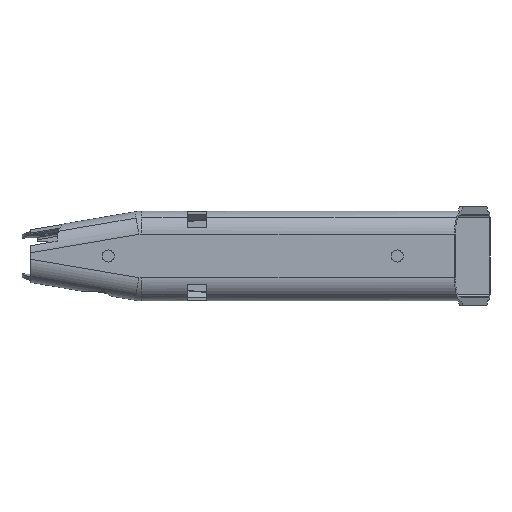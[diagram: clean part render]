
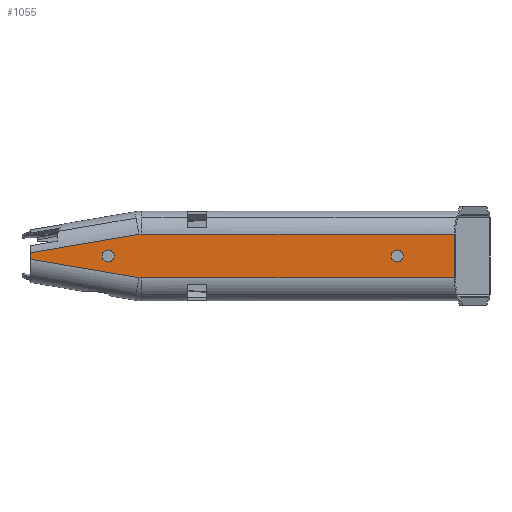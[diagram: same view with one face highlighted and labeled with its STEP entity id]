
A CAD part, left-side view. The second image highlights one B-rep face of the part: STEP entity #1055.
In plain terms, the highlighted planar face has unit normal (-1, 0, 0).
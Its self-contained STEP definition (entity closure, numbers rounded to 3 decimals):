
#151 = VECTOR ( 'NONE', #8540, 1000. ) ;
#191 = CARTESIAN_POINT ( 'NONE',  ( -16.053, -44.915, -5.429 ) ) ;
#270 = CARTESIAN_POINT ( 'NONE',  ( -16.053, 31.63, 5.247 ) ) ;
#440 = CARTESIAN_POINT ( 'NONE',  ( -16.053, 57.866, -5.429 ) ) ;
#818 = VECTOR ( 'NONE', #34573, 1000. ) ;
#1055 = ADVANCED_FACE ( 'NONE', ( #5729, #20576, #27072 ), #24698, .T. ) ;
#3311 = CARTESIAN_POINT ( 'NONE',  ( -16.053, 31.194, -5.302 ) ) ;
#4048 = EDGE_LOOP ( 'NONE', ( #18662, #35163 ) ) ;
#4184 = CARTESIAN_POINT ( 'NONE',  ( -16.053, 39.095, 0. ) ) ;
#4232 = CARTESIAN_POINT ( 'NONE',  ( -16.053, 30.974, 5.302 ) ) ;
#4390 = AXIS2_PLACEMENT_3D ( 'NONE', #7993, #7871, #30246 ) ;
#4706 = EDGE_CURVE ( 'NONE', #16376, #8779, #5169, .T. ) ;
#5014 = AXIS2_PLACEMENT_3D ( 'NONE', #4184, #23674, #6988 ) ;
#5169 = LINE ( 'NONE', #6656, #18212 ) ;
#5729 = FACE_OUTER_BOUND ( 'NONE', #26580, .T. ) ;
#6224 = CARTESIAN_POINT ( 'NONE',  ( -16.053, 31.413, 5.284 ) ) ;
#6656 = CARTESIAN_POINT ( 'NONE',  ( -16.053, 0., -5.302 ) ) ;
#6811 = ORIENTED_EDGE ( 'NONE', *, *, #25889, .F. ) ;
#6988 = DIRECTION ( 'NONE',  ( 0., 0., -1. ) ) ;
#7106 = CARTESIAN_POINT ( 'NONE',  ( -16.053, -30.983, -1.46 ) ) ;
#7265 = EDGE_CURVE ( 'NONE', #20646, #34797, #15037, .T. ) ;
#7276 = VERTEX_POINT ( 'NONE', #12723 ) ;
#7554 = LINE ( 'NONE', #28000, #151 ) ;
#7871 = DIRECTION ( 'NONE',  ( -1., 0., 0. ) ) ;
#7993 = CARTESIAN_POINT ( 'NONE',  ( -16.053, 0., -10.858 ) ) ;
#8221 = LINE ( 'NONE', #31768, #818 ) ;
#8540 = DIRECTION ( 'NONE',  ( 0., 0.986, 0.168 ) ) ;
#8707 = CARTESIAN_POINT ( 'NONE',  ( -16.053, -30.983, 0. ) ) ;
#8779 = VERTEX_POINT ( 'NONE', #25829 ) ;
#8908 = CARTESIAN_POINT ( 'NONE',  ( -16.053, 30.974, -5.302 ) ) ;
#9439 = VERTEX_POINT ( 'NONE', #4232 ) ;
#10057 = CIRCLE ( 'NONE', #20218, 1.46 ) ;
#10265 = VECTOR ( 'NONE', #24914, 1000. ) ;
#10284 = CARTESIAN_POINT ( 'NONE',  ( -16.053, -44.915, 5.302 ) ) ;
#10829 = LINE ( 'NONE', #191, #25614 ) ;
#11109 = VERTEX_POINT ( 'NONE', #20413 ) ;
#11409 = LINE ( 'NONE', #440, #25327 ) ;
#11528 = DIRECTION ( 'NONE',  ( 0., 0., -1. ) ) ;
#11565 = EDGE_CURVE ( 'NONE', #11109, #15018, #7554, .T. ) ;
#11848 = CARTESIAN_POINT ( 'NONE',  ( -16.053, 31.194, 5.302 ) ) ;
#12723 = CARTESIAN_POINT ( 'NONE',  ( -16.053, 57.866, 0.778 ) ) ;
#12824 = DIRECTION ( 'NONE',  ( 1., 0., 0. ) ) ;
#12900 = VERTEX_POINT ( 'NONE', #18799 ) ;
#13856 = EDGE_CURVE ( 'NONE', #34797, #20646, #34515, .T. ) ;
#14359 = DIRECTION ( 'NONE',  ( 0., 0., -1. ) ) ;
#14445 = EDGE_CURVE ( 'NONE', #7276, #15018, #11409, .T. ) ;
#14505 = DIRECTION ( 'NONE',  ( 1., 0., 0. ) ) ;
#14524 = CARTESIAN_POINT ( 'NONE',  ( -16.053, 31.413, -5.284 ) ) ;
#15018 = VERTEX_POINT ( 'NONE', #16203 ) ;
#15037 = CIRCLE ( 'NONE', #5014, 1.46 ) ;
#16203 = CARTESIAN_POINT ( 'NONE',  ( -16.053, 57.866, -0.778 ) ) ;
#16376 = VERTEX_POINT ( 'NONE', #33112 ) ;
#17141 = EDGE_CURVE ( 'NONE', #16376, #21055, #10829, .T. ) ;
#17532 = VERTEX_POINT ( 'NONE', #270 ) ;
#17955 = ORIENTED_EDGE ( 'NONE', *, *, #7265, .T. ) ;
#18212 = VECTOR ( 'NONE', #23478, 1000. ) ;
#18280 = AXIS2_PLACEMENT_3D ( 'NONE', #8707, #28159, #11528 ) ;
#18595 = EDGE_LOOP ( 'NONE', ( #17955, #22829 ) ) ;
#18662 = ORIENTED_EDGE ( 'NONE', *, *, #22969, .T. ) ;
#18799 = CARTESIAN_POINT ( 'NONE',  ( -16.053, -30.983, 1.461 ) ) ;
#19249 = ORIENTED_EDGE ( 'NONE', *, *, #11565, .F. ) ;
#19695 = DIRECTION ( 'NONE',  ( 0., 0., 1. ) ) ;
#20218 = AXIS2_PLACEMENT_3D ( 'NONE', #29430, #12824, #32258 ) ;
#20413 = CARTESIAN_POINT ( 'NONE',  ( -16.053, 31.63, -5.247 ) ) ;
#20576 = FACE_BOUND ( 'NONE', #18595, .T. ) ;
#20646 = VERTEX_POINT ( 'NONE', #23236 ) ;
#21014 = ORIENTED_EDGE ( 'NONE', *, *, #31857, .F. ) ;
#21055 = VERTEX_POINT ( 'NONE', #10284 ) ;
#21156 = ORIENTED_EDGE ( 'NONE', *, *, #24357, .F. ) ;
#22796 = CARTESIAN_POINT ( 'NONE',  ( -16.053, 31.63, 5.247 ) ) ;
#22829 = ORIENTED_EDGE ( 'NONE', *, *, #13856, .T. ) ;
#22969 = EDGE_CURVE ( 'NONE', #32157, #12900, #10057, .T. ) ;
#23236 = CARTESIAN_POINT ( 'NONE',  ( -16.053, 39.095, -1.46 ) ) ;
#23478 = DIRECTION ( 'NONE',  ( 0., 1., 0. ) ) ;
#23674 = DIRECTION ( 'NONE',  ( 1., 0., 0. ) ) ;
#24251 = ORIENTED_EDGE ( 'NONE', *, *, #14445, .T. ) ;
#24306 = ORIENTED_EDGE ( 'NONE', *, *, #4706, .F. ) ;
#24357 = EDGE_CURVE ( 'NONE', #7276, #17532, #8221, .T. ) ;
#24698 = PLANE ( 'NONE',  #4390 ) ;
#24914 = DIRECTION ( 'NONE',  ( 0., -1., 0. ) ) ;
#25078 = LINE ( 'NONE', #27694, #10265 ) ;
#25327 = VECTOR ( 'NONE', #14359, 1000. ) ;
#25474 =( BOUNDED_CURVE ( )  B_SPLINE_CURVE ( 3, ( #22796, #6224, #11848, #31297 ),
 .UNSPECIFIED., .F., .F. ) 
 B_SPLINE_CURVE_WITH_KNOTS ( ( 4, 4 ),
 ( 1.396, 1.571 ),
 .UNSPECIFIED. ) 
 CURVE ( )  GEOMETRIC_REPRESENTATION_ITEM ( )  RATIONAL_B_SPLINE_CURVE ( ( 1., 0.997, 0.997, 1. ) ) 
 REPRESENTATION_ITEM ( '' )  );
#25614 = VECTOR ( 'NONE', #19695, 1000. ) ;
#25829 = CARTESIAN_POINT ( 'NONE',  ( -16.053, 30.974, -5.302 ) ) ;
#25889 = EDGE_CURVE ( 'NONE', #17532, #9439, #25474, .T. ) ;
#26566 = ORIENTED_EDGE ( 'NONE', *, *, #17141, .T. ) ;
#26580 = EDGE_LOOP ( 'NONE', ( #32883, #24306, #26566, #21014, #6811, #21156, #24251, #19249 ) ) ;
#26802 = AXIS2_PLACEMENT_3D ( 'NONE', #31152, #14505, #33963 ) ;
#27072 = FACE_BOUND ( 'NONE', #4048, .T. ) ;
#27520 =( BOUNDED_CURVE ( )  B_SPLINE_CURVE ( 3, ( #8908, #3311, #14524, #33982 ),
 .UNSPECIFIED., .F., .F. ) 
 B_SPLINE_CURVE_WITH_KNOTS ( ( 4, 4 ),
 ( 4.712, 4.887 ),
 .UNSPECIFIED. ) 
 CURVE ( )  GEOMETRIC_REPRESENTATION_ITEM ( )  RATIONAL_B_SPLINE_CURVE ( ( 1., 0.997, 0.997, 1. ) ) 
 REPRESENTATION_ITEM ( '' )  );
#27694 = CARTESIAN_POINT ( 'NONE',  ( -16.053, 0., 5.302 ) ) ;
#27736 = CIRCLE ( 'NONE', #18280, 1.46 ) ;
#28000 = CARTESIAN_POINT ( 'NONE',  ( -16.053, 9.416, -9.03 ) ) ;
#28159 = DIRECTION ( 'NONE',  ( 1., 0., 0. ) ) ;
#29430 = CARTESIAN_POINT ( 'NONE',  ( -16.053, -30.983, 0. ) ) ;
#30246 = DIRECTION ( 'NONE',  ( 0., 0., 1. ) ) ;
#30473 = EDGE_CURVE ( 'NONE', #12900, #32157, #27736, .T. ) ;
#30809 = CARTESIAN_POINT ( 'NONE',  ( -16.053, 39.095, 1.461 ) ) ;
#31152 = CARTESIAN_POINT ( 'NONE',  ( -16.053, 39.095, 0. ) ) ;
#31297 = CARTESIAN_POINT ( 'NONE',  ( -16.053, 30.974, 5.302 ) ) ;
#31768 = CARTESIAN_POINT ( 'NONE',  ( -16.053, 25.825, 6.235 ) ) ;
#31857 = EDGE_CURVE ( 'NONE', #9439, #21055, #25078, .T. ) ;
#32157 = VERTEX_POINT ( 'NONE', #7106 ) ;
#32258 = DIRECTION ( 'NONE',  ( 0., 0., -1. ) ) ;
#32883 = ORIENTED_EDGE ( 'NONE', *, *, #35738, .F. ) ;
#33112 = CARTESIAN_POINT ( 'NONE',  ( -16.053, -44.915, -5.302 ) ) ;
#33963 = DIRECTION ( 'NONE',  ( 0., 0., -1. ) ) ;
#33982 = CARTESIAN_POINT ( 'NONE',  ( -16.053, 31.63, -5.247 ) ) ;
#34515 = CIRCLE ( 'NONE', #26802, 1.46 ) ;
#34573 = DIRECTION ( 'NONE',  ( 0., -0.986, 0.168 ) ) ;
#34797 = VERTEX_POINT ( 'NONE', #30809 ) ;
#35163 = ORIENTED_EDGE ( 'NONE', *, *, #30473, .T. ) ;
#35738 = EDGE_CURVE ( 'NONE', #8779, #11109, #27520, .T. ) ;
